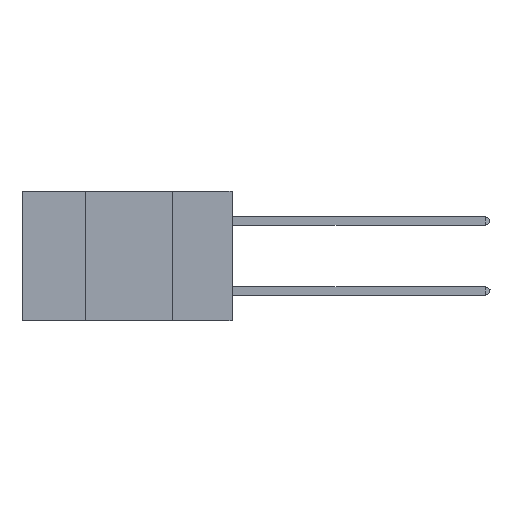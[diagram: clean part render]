
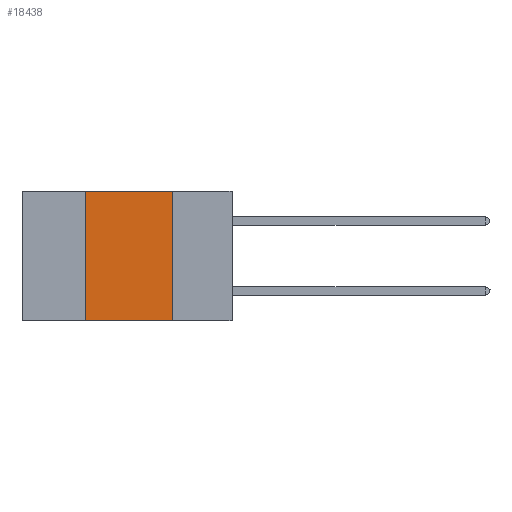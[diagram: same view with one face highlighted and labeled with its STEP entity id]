
A CAD part, left-side view. The second image highlights one B-rep face of the part: STEP entity #18438.
In plain terms, the highlighted planar face has unit normal (-1, 0, 0).
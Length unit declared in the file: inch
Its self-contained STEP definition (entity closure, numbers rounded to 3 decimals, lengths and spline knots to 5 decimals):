
#127 = LINE ( 'NONE', #9702, #8959 ) ;
#325 = DIRECTION ( 'NONE',  ( 0., 0., -1. ) ) ;
#521 = CARTESIAN_POINT ( 'NONE',  ( 0., 0.17, 0. ) ) ;
#1429 = CARTESIAN_POINT ( 'NONE',  ( 0., 0.42, 0. ) ) ;
#1532 = VERTEX_POINT ( 'NONE', #18509 ) ;
#1666 = LINE ( 'NONE', #6117, #5449 ) ;
#2983 = PLANE ( 'NONE',  #15814 ) ;
#3179 = ORIENTED_EDGE ( 'NONE', *, *, #11295, .F. ) ;
#4564 = DIRECTION ( 'NONE',  ( 0., 0., 1. ) ) ;
#5029 = EDGE_CURVE ( 'NONE', #6561, #6925, #127, .T. ) ;
#5201 = ORIENTED_EDGE ( 'NONE', *, *, #17474, .F. ) ;
#5449 = VECTOR ( 'NONE', #4564, 39.37008 ) ;
#6117 = CARTESIAN_POINT ( 'NONE',  ( 0., 0.42, 0. ) ) ;
#6166 = CARTESIAN_POINT ( 'NONE',  ( 0., 0.6, 0. ) ) ;
#6210 = VECTOR ( 'NONE', #12191, 39.37008 ) ;
#6561 = VERTEX_POINT ( 'NONE', #521 ) ;
#6925 = VERTEX_POINT ( 'NONE', #19613 ) ;
#7188 = VECTOR ( 'NONE', #10393, 39.37008 ) ;
#8959 = VECTOR ( 'NONE', #325, 39.37008 ) ;
#9205 = DIRECTION ( 'NONE',  ( 0., 0., -1. ) ) ;
#9702 = CARTESIAN_POINT ( 'NONE',  ( 0., 0.17, 0. ) ) ;
#10393 = DIRECTION ( 'NONE',  ( 0., -1., 0. ) ) ;
#10476 = EDGE_CURVE ( 'NONE', #1532, #6925, #14715, .T. ) ;
#10691 = CARTESIAN_POINT ( 'NONE',  ( 0., 0.6, 0. ) ) ;
#10708 = LINE ( 'NONE', #10691, #6210 ) ;
#11295 = EDGE_CURVE ( 'NONE', #18444, #6561, #10708, .T. ) ;
#12191 = DIRECTION ( 'NONE',  ( 0., -1., 0. ) ) ;
#12481 = FACE_OUTER_BOUND ( 'NONE', #14467, .T. ) ;
#14467 = EDGE_LOOP ( 'NONE', ( #18349, #3179, #5201, #17421 ) ) ;
#14715 = LINE ( 'NONE', #16330, #7188 ) ;
#15814 = AXIS2_PLACEMENT_3D ( 'NONE', #6166, #18164, #9205 ) ;
#16330 = CARTESIAN_POINT ( 'NONE',  ( 0., 0.6, -0.37 ) ) ;
#17421 = ORIENTED_EDGE ( 'NONE', *, *, #10476, .T. ) ;
#17474 = EDGE_CURVE ( 'NONE', #1532, #18444, #1666, .T. ) ;
#18164 = DIRECTION ( 'NONE',  ( 1., 0., 0. ) ) ;
#18349 = ORIENTED_EDGE ( 'NONE', *, *, #5029, .F. ) ;
#18438 = ADVANCED_FACE ( 'NONE', ( #12481 ), #2983, .F. ) ;
#18444 = VERTEX_POINT ( 'NONE', #1429 ) ;
#18509 = CARTESIAN_POINT ( 'NONE',  ( 0., 0.42, -0.37 ) ) ;
#19613 = CARTESIAN_POINT ( 'NONE',  ( 0., 0.17, -0.37 ) ) ;
